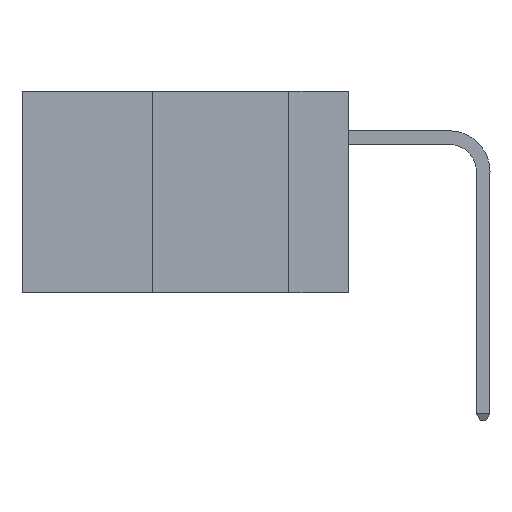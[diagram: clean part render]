
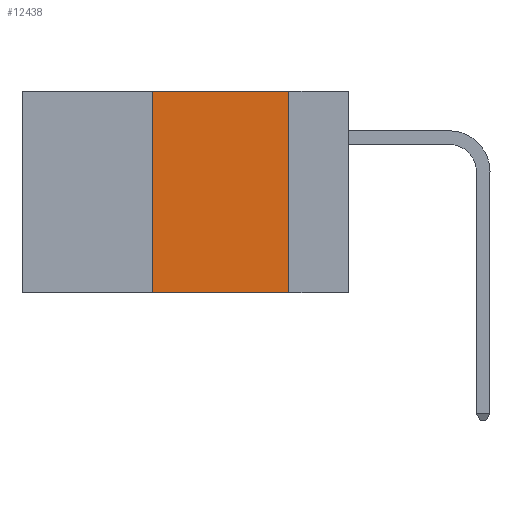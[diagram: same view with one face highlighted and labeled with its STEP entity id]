
A CAD part, left-side view. The second image highlights one B-rep face of the part: STEP entity #12438.
In plain terms, the highlighted planar face has unit normal (-1, 0, 0).
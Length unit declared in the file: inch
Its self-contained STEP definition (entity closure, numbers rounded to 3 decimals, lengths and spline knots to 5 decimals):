
#535 = VERTEX_POINT ( 'NONE', #4671 ) ;
#1013 = VECTOR ( 'NONE', #7144, 39.37008 ) ;
#1561 = CARTESIAN_POINT ( 'NONE',  ( 0., 0.11, 0. ) ) ;
#1839 = PLANE ( 'NONE',  #15657 ) ;
#2173 = LINE ( 'NONE', #1561, #21157 ) ;
#2429 = EDGE_LOOP ( 'NONE', ( #21323, #10818, #12508, #20344 ) ) ;
#3262 = VERTEX_POINT ( 'NONE', #12996 ) ;
#3599 = CARTESIAN_POINT ( 'NONE',  ( 0., 0.6, 0. ) ) ;
#4266 = VERTEX_POINT ( 'NONE', #19551 ) ;
#4282 = VECTOR ( 'NONE', #10851, 39.37008 ) ;
#4671 = CARTESIAN_POINT ( 'NONE',  ( 0., 0.11, 0. ) ) ;
#5434 = CARTESIAN_POINT ( 'NONE',  ( 0., 0.6, -0.37 ) ) ;
#6875 = LINE ( 'NONE', #19683, #15535 ) ;
#6907 = EDGE_CURVE ( 'NONE', #4266, #3262, #20583, .T. ) ;
#7120 = DIRECTION ( 'NONE',  ( 0., 0., -1. ) ) ;
#7144 = DIRECTION ( 'NONE',  ( 0., -1., 0. ) ) ;
#8853 = LINE ( 'NONE', #15986, #4282 ) ;
#10712 = VERTEX_POINT ( 'NONE', #14794 ) ;
#10818 = ORIENTED_EDGE ( 'NONE', *, *, #15299, .F. ) ;
#10851 = DIRECTION ( 'NONE',  ( 0., -1., 0. ) ) ;
#10886 = FACE_OUTER_BOUND ( 'NONE', #2429, .T. ) ;
#11061 = DIRECTION ( 'NONE',  ( 0., 0., 1. ) ) ;
#12438 = ADVANCED_FACE ( 'NONE', ( #10886 ), #1839, .F. ) ;
#12508 = ORIENTED_EDGE ( 'NONE', *, *, #21526, .F. ) ;
#12996 = CARTESIAN_POINT ( 'NONE',  ( 0., 0.11, -0.37 ) ) ;
#14794 = CARTESIAN_POINT ( 'NONE',  ( 0., 0.36, 0. ) ) ;
#15299 = EDGE_CURVE ( 'NONE', #10712, #535, #8853, .T. ) ;
#15535 = VECTOR ( 'NONE', #11061, 39.37008 ) ;
#15657 = AXIS2_PLACEMENT_3D ( 'NONE', #3599, #17494, #7120 ) ;
#15986 = CARTESIAN_POINT ( 'NONE',  ( 0., 0.6, 0. ) ) ;
#16532 = EDGE_CURVE ( 'NONE', #535, #3262, #2173, .T. ) ;
#17494 = DIRECTION ( 'NONE',  ( 1., 0., 0. ) ) ;
#19551 = CARTESIAN_POINT ( 'NONE',  ( 0., 0.36, -0.37 ) ) ;
#19683 = CARTESIAN_POINT ( 'NONE',  ( 0., 0.36, 0. ) ) ;
#20344 = ORIENTED_EDGE ( 'NONE', *, *, #6907, .T. ) ;
#20583 = LINE ( 'NONE', #5434, #1013 ) ;
#21157 = VECTOR ( 'NONE', #22296, 39.37008 ) ;
#21323 = ORIENTED_EDGE ( 'NONE', *, *, #16532, .F. ) ;
#21526 = EDGE_CURVE ( 'NONE', #4266, #10712, #6875, .T. ) ;
#22296 = DIRECTION ( 'NONE',  ( 0., 0., -1. ) ) ;
